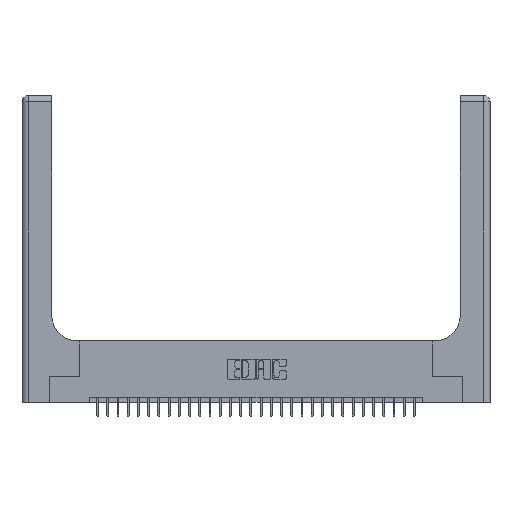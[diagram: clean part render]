
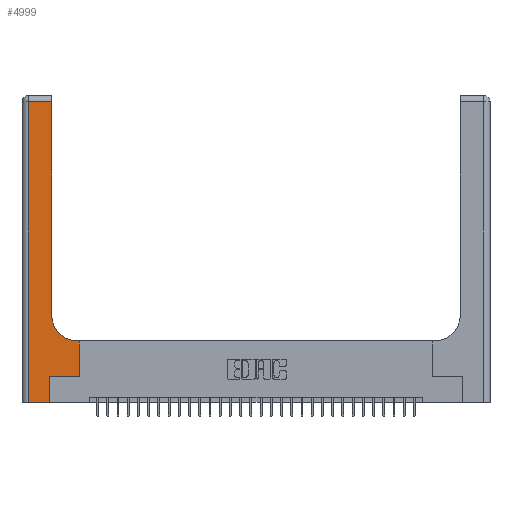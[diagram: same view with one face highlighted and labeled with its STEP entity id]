
A CAD part, top view. The second image highlights one B-rep face of the part: STEP entity #4999.
In plain terms, the highlighted planar face has unit normal (0, 0, 1).
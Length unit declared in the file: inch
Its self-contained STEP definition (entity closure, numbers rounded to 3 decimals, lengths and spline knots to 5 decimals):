
#686 = DIRECTION ( 'NONE',  ( 0., 1., 0. ) ) ;
#1789 = VERTEX_POINT ( 'NONE', #10602 ) ;
#2252 = CARTESIAN_POINT ( 'NONE',  ( 0.2915, 0.6, 0.37 ) ) ;
#3122 = LINE ( 'NONE', #18074, #29169 ) ;
#3819 = DIRECTION ( 'NONE',  ( -1., 0., 0. ) ) ;
#4258 = EDGE_CURVE ( 'NONE', #18259, #28006, #6358, .T. ) ;
#4334 = LINE ( 'NONE', #21221, #26968 ) ;
#4999 = ADVANCED_FACE ( 'NONE', ( #28083 ), #13199, .F. ) ;
#5224 = ORIENTED_EDGE ( 'NONE', *, *, #28719, .T. ) ;
#5572 = EDGE_CURVE ( 'NONE', #15688, #13781, #27315, .T. ) ;
#6217 = LINE ( 'NONE', #16070, #28248 ) ;
#6358 = LINE ( 'NONE', #30767, #15003 ) ;
#7668 = VECTOR ( 'NONE', #25178, 39.37008 ) ;
#8039 = CARTESIAN_POINT ( 'NONE',  ( 0.06, 2.94, 0.37 ) ) ;
#8101 = ORIENTED_EDGE ( 'NONE', *, *, #19642, .T. ) ;
#8355 = DIRECTION ( 'NONE',  ( -1., 0., 0. ) ) ;
#8550 = LINE ( 'NONE', #20920, #19463 ) ;
#9194 = CARTESIAN_POINT ( 'NONE',  ( 0.5585, 0.25, 0.37 ) ) ;
#9844 = ORIENTED_EDGE ( 'NONE', *, *, #5572, .T. ) ;
#10602 = CARTESIAN_POINT ( 'NONE',  ( 0.2915, 2.94, 0.37 ) ) ;
#11063 = DIRECTION ( 'NONE',  ( 0., 1., 0. ) ) ;
#11679 = EDGE_CURVE ( 'NONE', #14262, #18259, #26043, .T. ) ;
#12064 = VECTOR ( 'NONE', #13732, 39.37008 ) ;
#12094 = LINE ( 'NONE', #2252, #25040 ) ;
#13088 = CARTESIAN_POINT ( 'NONE',  ( 0.269, 0.25, 0.37 ) ) ;
#13199 = PLANE ( 'NONE',  #25743 ) ;
#13519 = EDGE_CURVE ( 'NONE', #27180, #30112, #4334, .T. ) ;
#13732 = DIRECTION ( 'NONE',  ( 1., 0., 0. ) ) ;
#13781 = VERTEX_POINT ( 'NONE', #24715 ) ;
#13898 = CARTESIAN_POINT ( 'NONE',  ( 0.5585, 0.6, 0.37 ) ) ;
#14262 = VERTEX_POINT ( 'NONE', #23177 ) ;
#15003 = VECTOR ( 'NONE', #11063, 39.37008 ) ;
#15294 = DIRECTION ( 'NONE',  ( 0., 0., -1. ) ) ;
#15688 = VERTEX_POINT ( 'NONE', #21962 ) ;
#15929 = CARTESIAN_POINT ( 'NONE',  ( 0., 3., 0.37 ) ) ;
#16070 = CARTESIAN_POINT ( 'NONE',  ( 0., 2.94, 0.37 ) ) ;
#16275 = ORIENTED_EDGE ( 'NONE', *, *, #4258, .T. ) ;
#16366 = DIRECTION ( 'NONE',  ( 1., 0., 0. ) ) ;
#16722 = DIRECTION ( 'NONE',  ( 1., 0., 0. ) ) ;
#16880 = EDGE_CURVE ( 'NONE', #28006, #15688, #12094, .T. ) ;
#17245 = ORIENTED_EDGE ( 'NONE', *, *, #11679, .T. ) ;
#17509 = EDGE_CURVE ( 'NONE', #13781, #1789, #3122, .T. ) ;
#17589 = AXIS2_PLACEMENT_3D ( 'NONE', #21477, #21324, #16366 ) ;
#18074 = CARTESIAN_POINT ( 'NONE',  ( 0.2915, 3., 0.37 ) ) ;
#18259 = VERTEX_POINT ( 'NONE', #9194 ) ;
#18908 = ORIENTED_EDGE ( 'NONE', *, *, #17509, .T. ) ;
#19463 = VECTOR ( 'NONE', #23164, 39.37008 ) ;
#19642 = EDGE_CURVE ( 'NONE', #30112, #14262, #8550, .T. ) ;
#20920 = CARTESIAN_POINT ( 'NONE',  ( 0.269, 0., 0.37 ) ) ;
#21221 = CARTESIAN_POINT ( 'NONE',  ( 0., 0., 0.37 ) ) ;
#21324 = DIRECTION ( 'NONE',  ( 0., 0., -1. ) ) ;
#21477 = CARTESIAN_POINT ( 'NONE',  ( 0.5415, 0.85, 0.37 ) ) ;
#21962 = CARTESIAN_POINT ( 'NONE',  ( 0.5415, 0.6, 0.37 ) ) ;
#23164 = DIRECTION ( 'NONE',  ( 0., 1., 0. ) ) ;
#23177 = CARTESIAN_POINT ( 'NONE',  ( 0.269, 0.25, 0.37 ) ) ;
#23824 = EDGE_LOOP ( 'NONE', ( #18908, #26937, #5224, #27554, #8101, #17245, #16275, #30890, #9844 ) ) ;
#24092 = DIRECTION ( 'NONE',  ( -1., 0., 0. ) ) ;
#24708 = CARTESIAN_POINT ( 'NONE',  ( 0.06, 3., 0.37 ) ) ;
#24715 = CARTESIAN_POINT ( 'NONE',  ( 0.2915, 0.85, 0.37 ) ) ;
#25040 = VECTOR ( 'NONE', #24092, 39.37008 ) ;
#25178 = DIRECTION ( 'NONE',  ( 0., -1., 0. ) ) ;
#25653 = CARTESIAN_POINT ( 'NONE',  ( 0.269, 0., 0.37 ) ) ;
#25743 = AXIS2_PLACEMENT_3D ( 'NONE', #15929, #15294, #8355 ) ;
#26043 = LINE ( 'NONE', #13088, #12064 ) ;
#26937 = ORIENTED_EDGE ( 'NONE', *, *, #30221, .T. ) ;
#26968 = VECTOR ( 'NONE', #16722, 39.37008 ) ;
#27106 = CARTESIAN_POINT ( 'NONE',  ( 0.06, 0., 0.37 ) ) ;
#27112 = LINE ( 'NONE', #24708, #7668 ) ;
#27180 = VERTEX_POINT ( 'NONE', #27106 ) ;
#27315 = CIRCLE ( 'NONE', #17589, 0.25 ) ;
#27554 = ORIENTED_EDGE ( 'NONE', *, *, #13519, .T. ) ;
#28006 = VERTEX_POINT ( 'NONE', #13898 ) ;
#28083 = FACE_OUTER_BOUND ( 'NONE', #23824, .T. ) ;
#28248 = VECTOR ( 'NONE', #3819, 39.37008 ) ;
#28719 = EDGE_CURVE ( 'NONE', #29580, #27180, #27112, .T. ) ;
#29169 = VECTOR ( 'NONE', #686, 39.37008 ) ;
#29580 = VERTEX_POINT ( 'NONE', #8039 ) ;
#30112 = VERTEX_POINT ( 'NONE', #25653 ) ;
#30221 = EDGE_CURVE ( 'NONE', #1789, #29580, #6217, .T. ) ;
#30767 = CARTESIAN_POINT ( 'NONE',  ( 0.5585, 0.25, 0.37 ) ) ;
#30890 = ORIENTED_EDGE ( 'NONE', *, *, #16880, .T. ) ;
